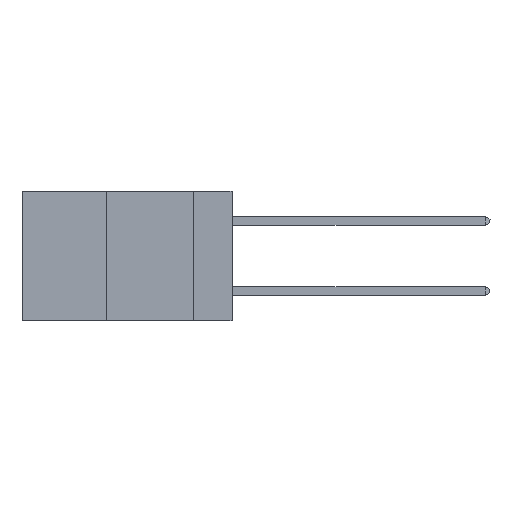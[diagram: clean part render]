
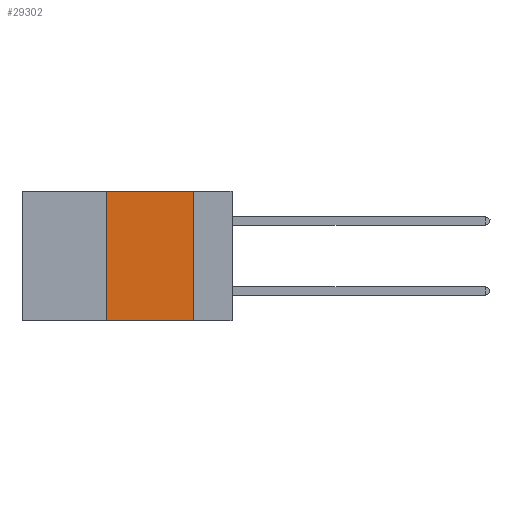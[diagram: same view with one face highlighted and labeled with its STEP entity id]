
A CAD part, left-side view. The second image highlights one B-rep face of the part: STEP entity #29302.
In plain terms, the highlighted planar face has unit normal (-1, 0, 0).
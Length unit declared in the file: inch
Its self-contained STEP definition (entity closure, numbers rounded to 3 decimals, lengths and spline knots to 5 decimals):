
#1638 = VECTOR ( 'NONE', #11178, 39.37008 ) ;
#1772 = CARTESIAN_POINT ( 'NONE',  ( 0., 0.36, -0.37 ) ) ;
#3510 = DIRECTION ( 'NONE',  ( 0., 0., -1. ) ) ;
#4403 = DIRECTION ( 'NONE',  ( 0., -1., 0. ) ) ;
#7532 = VECTOR ( 'NONE', #25409, 39.37008 ) ;
#9516 = VERTEX_POINT ( 'NONE', #33670 ) ;
#9892 = AXIS2_PLACEMENT_3D ( 'NONE', #45242, #25105, #3510 ) ;
#11178 = DIRECTION ( 'NONE',  ( 0., 0., 1. ) ) ;
#11448 = LINE ( 'NONE', #35564, #1638 ) ;
#11831 = EDGE_CURVE ( 'NONE', #44448, #30543, #26244, .T. ) ;
#13425 = CARTESIAN_POINT ( 'NONE',  ( 0., 0.11, 0. ) ) ;
#14417 = PLANE ( 'NONE',  #9892 ) ;
#15800 = VERTEX_POINT ( 'NONE', #21965 ) ;
#20383 = FACE_OUTER_BOUND ( 'NONE', #42320, .T. ) ;
#20544 = DIRECTION ( 'NONE',  ( 0., 0., -1. ) ) ;
#21965 = CARTESIAN_POINT ( 'NONE',  ( 0., 0.36, 0. ) ) ;
#23080 = LINE ( 'NONE', #13425, #30110 ) ;
#25105 = DIRECTION ( 'NONE',  ( 1., 0., 0. ) ) ;
#25409 = DIRECTION ( 'NONE',  ( 0., -1., 0. ) ) ;
#26244 = LINE ( 'NONE', #39323, #40944 ) ;
#29302 = ADVANCED_FACE ( 'NONE', ( #20383 ), #14417, .F. ) ;
#29332 = ORIENTED_EDGE ( 'NONE', *, *, #43878, .F. ) ;
#30110 = VECTOR ( 'NONE', #20544, 39.37008 ) ;
#30543 = VERTEX_POINT ( 'NONE', #33126 ) ;
#32266 = CARTESIAN_POINT ( 'NONE',  ( 0., 0.6, 0. ) ) ;
#33126 = CARTESIAN_POINT ( 'NONE',  ( 0., 0.11, -0.37 ) ) ;
#33670 = CARTESIAN_POINT ( 'NONE',  ( 0., 0.11, 0. ) ) ;
#35564 = CARTESIAN_POINT ( 'NONE',  ( 0., 0.36, 0. ) ) ;
#39323 = CARTESIAN_POINT ( 'NONE',  ( 0., 0.6, -0.37 ) ) ;
#39624 = ORIENTED_EDGE ( 'NONE', *, *, #44132, .F. ) ;
#40333 = ORIENTED_EDGE ( 'NONE', *, *, #11831, .T. ) ;
#40429 = ORIENTED_EDGE ( 'NONE', *, *, #42806, .F. ) ;
#40944 = VECTOR ( 'NONE', #4403, 39.37008 ) ;
#42320 = EDGE_LOOP ( 'NONE', ( #29332, #40429, #39624, #40333 ) ) ;
#42806 = EDGE_CURVE ( 'NONE', #15800, #9516, #43338, .T. ) ;
#43338 = LINE ( 'NONE', #32266, #7532 ) ;
#43878 = EDGE_CURVE ( 'NONE', #9516, #30543, #23080, .T. ) ;
#44132 = EDGE_CURVE ( 'NONE', #44448, #15800, #11448, .T. ) ;
#44448 = VERTEX_POINT ( 'NONE', #1772 ) ;
#45242 = CARTESIAN_POINT ( 'NONE',  ( 0., 0.6, 0. ) ) ;
